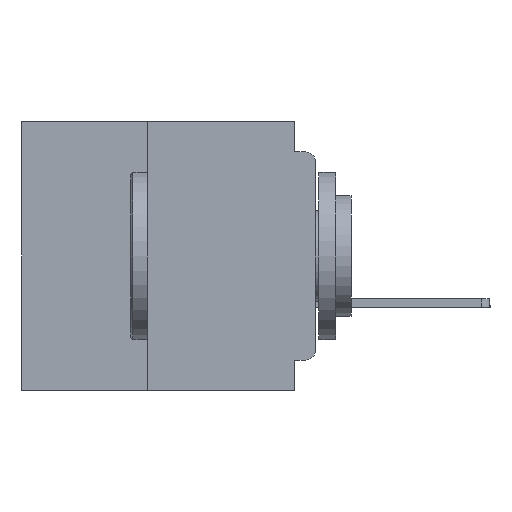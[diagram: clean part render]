
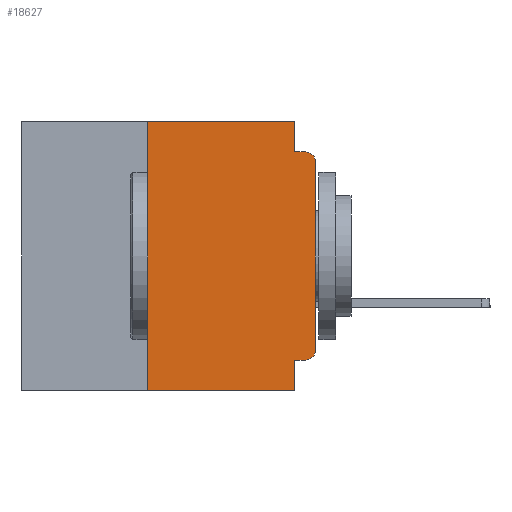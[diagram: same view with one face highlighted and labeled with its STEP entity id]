
A CAD part, left-side view. The second image highlights one B-rep face of the part: STEP entity #18627.
In plain terms, the highlighted planar face has unit normal (-1, 0, 0).
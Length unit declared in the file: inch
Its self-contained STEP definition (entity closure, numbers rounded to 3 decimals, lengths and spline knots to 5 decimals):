
#276 = EDGE_CURVE ( 'NONE', #13432, #35435, #7282, .T. ) ;
#452 = VERTEX_POINT ( 'NONE', #28619 ) ;
#608 = VECTOR ( 'NONE', #24151, 39.37008 ) ;
#1027 = DIRECTION ( 'NONE',  ( 0., 0., -1. ) ) ;
#1033 = CARTESIAN_POINT ( 'NONE',  ( 0., 0.031, -0.355 ) ) ;
#1709 = CARTESIAN_POINT ( 'NONE',  ( 0., 0.031, 0. ) ) ;
#1861 = DIRECTION ( 'NONE',  ( 0., 0., -1. ) ) ;
#2260 = CARTESIAN_POINT ( 'NONE',  ( 0., 0.031, -0.4 ) ) ;
#2428 = VECTOR ( 'NONE', #19470, 39.37008 ) ;
#3715 = CARTESIAN_POINT ( 'NONE',  ( 0., 0.031, 0. ) ) ;
#4009 = LINE ( 'NONE', #33039, #11389 ) ;
#4028 = CIRCLE ( 'NONE', #7651, 0.015 ) ;
#4280 = ORIENTED_EDGE ( 'NONE', *, *, #9184, .T. ) ;
#4414 = VERTEX_POINT ( 'NONE', #18378 ) ;
#5037 = ORIENTED_EDGE ( 'NONE', *, *, #34478, .F. ) ;
#5732 = VECTOR ( 'NONE', #16223, 39.37008 ) ;
#5984 = CARTESIAN_POINT ( 'NONE',  ( 0., 0.015, -0.06 ) ) ;
#7025 = FACE_OUTER_BOUND ( 'NONE', #15466, .T. ) ;
#7117 = LINE ( 'NONE', #10163, #608 ) ;
#7175 = VERTEX_POINT ( 'NONE', #1033 ) ;
#7191 = DIRECTION ( 'NONE',  ( 0., -1., 0. ) ) ;
#7282 = LINE ( 'NONE', #1709, #30344 ) ;
#7651 = AXIS2_PLACEMENT_3D ( 'NONE', #35040, #18512, #1861 ) ;
#8563 = ORIENTED_EDGE ( 'NONE', *, *, #30683, .T. ) ;
#8800 = DIRECTION ( 'NONE',  ( 0., 0., -1. ) ) ;
#8905 = CARTESIAN_POINT ( 'NONE',  ( 0., 0.25, 0. ) ) ;
#9120 = EDGE_CURVE ( 'NONE', #33688, #452, #34362, .T. ) ;
#9158 = EDGE_CURVE ( 'NONE', #35435, #24258, #26239, .T. ) ;
#9184 = EDGE_CURVE ( 'NONE', #33331, #33688, #4028, .T. ) ;
#9328 = PLANE ( 'NONE',  #16297 ) ;
#10163 = CARTESIAN_POINT ( 'NONE',  ( 0., 0., -0.355 ) ) ;
#10335 = AXIS2_PLACEMENT_3D ( 'NONE', #5984, #25486, #8800 ) ;
#10351 = ORIENTED_EDGE ( 'NONE', *, *, #21528, .F. ) ;
#11389 = VECTOR ( 'NONE', #22030, 39.37008 ) ;
#11803 = ORIENTED_EDGE ( 'NONE', *, *, #9120, .T. ) ;
#12261 = ORIENTED_EDGE ( 'NONE', *, *, #22802, .T. ) ;
#12277 = VECTOR ( 'NONE', #7191, 39.37008 ) ;
#12661 = CARTESIAN_POINT ( 'NONE',  ( 0., 0., 0. ) ) ;
#13092 = CARTESIAN_POINT ( 'NONE',  ( 0., 0.031, -0.045 ) ) ;
#13432 = VERTEX_POINT ( 'NONE', #3715 ) ;
#14575 = VERTEX_POINT ( 'NONE', #30294 ) ;
#14913 = DIRECTION ( 'NONE',  ( 1., 0., 0. ) ) ;
#15466 = EDGE_LOOP ( 'NONE', ( #11803, #12261, #21797, #28809, #5037, #20275, #8563, #17272, #10351, #4280 ) ) ;
#16223 = DIRECTION ( 'NONE',  ( 0., 0., -1. ) ) ;
#16297 = AXIS2_PLACEMENT_3D ( 'NONE', #28794, #14913, #34265 ) ;
#16672 = CARTESIAN_POINT ( 'NONE',  ( 0., 0.437, 0. ) ) ;
#17272 = ORIENTED_EDGE ( 'NONE', *, *, #22589, .F. ) ;
#18378 = CARTESIAN_POINT ( 'NONE',  ( 0., 0.25, -0.4 ) ) ;
#18385 = CARTESIAN_POINT ( 'NONE',  ( 0., 0., -0.045 ) ) ;
#18512 = DIRECTION ( 'NONE',  ( -1., 0., 0. ) ) ;
#18627 = ADVANCED_FACE ( 'NONE', ( #7025 ), #9328, .F. ) ;
#19470 = DIRECTION ( 'NONE',  ( 0., -1., 0. ) ) ;
#20275 = ORIENTED_EDGE ( 'NONE', *, *, #22684, .F. ) ;
#20718 = CARTESIAN_POINT ( 'NONE',  ( 0., 0.015, -0.045 ) ) ;
#20985 = CARTESIAN_POINT ( 'NONE',  ( 0., 0.437, -0.4 ) ) ;
#21100 = DIRECTION ( 'NONE',  ( 0., -1., 0. ) ) ;
#21391 = VECTOR ( 'NONE', #21100, 39.37008 ) ;
#21528 = EDGE_CURVE ( 'NONE', #33331, #7175, #7117, .T. ) ;
#21797 = ORIENTED_EDGE ( 'NONE', *, *, #9158, .F. ) ;
#22030 = DIRECTION ( 'NONE',  ( 0., 0., 1. ) ) ;
#22589 = EDGE_CURVE ( 'NONE', #7175, #14575, #27951, .T. ) ;
#22684 = EDGE_CURVE ( 'NONE', #4414, #26399, #4009, .T. ) ;
#22802 = EDGE_CURVE ( 'NONE', #452, #24258, #28359, .T. ) ;
#24151 = DIRECTION ( 'NONE',  ( 0., 1., 0. ) ) ;
#24258 = VERTEX_POINT ( 'NONE', #20718 ) ;
#25486 = DIRECTION ( 'NONE',  ( -1., 0., 0. ) ) ;
#25508 = LINE ( 'NONE', #16672, #2428 ) ;
#26239 = LINE ( 'NONE', #18385, #12277 ) ;
#26399 = VERTEX_POINT ( 'NONE', #8905 ) ;
#27112 = CARTESIAN_POINT ( 'NONE',  ( 0., 0., -0.34 ) ) ;
#27951 = LINE ( 'NONE', #2260, #5732 ) ;
#28359 = CIRCLE ( 'NONE', #10335, 0.015 ) ;
#28619 = CARTESIAN_POINT ( 'NONE',  ( 0., 0., -0.06 ) ) ;
#28794 = CARTESIAN_POINT ( 'NONE',  ( 0., 0.437, 0. ) ) ;
#28809 = ORIENTED_EDGE ( 'NONE', *, *, #276, .F. ) ;
#28820 = LINE ( 'NONE', #20985, #21391 ) ;
#30294 = CARTESIAN_POINT ( 'NONE',  ( 0., 0.031, -0.4 ) ) ;
#30344 = VECTOR ( 'NONE', #1027, 39.37008 ) ;
#30683 = EDGE_CURVE ( 'NONE', #4414, #14575, #28820, .T. ) ;
#32073 = DIRECTION ( 'NONE',  ( 0., 0., 1. ) ) ;
#32833 = CARTESIAN_POINT ( 'NONE',  ( 0., 0.015, -0.355 ) ) ;
#33039 = CARTESIAN_POINT ( 'NONE',  ( 0., 0.25, -0.4 ) ) ;
#33331 = VERTEX_POINT ( 'NONE', #32833 ) ;
#33688 = VERTEX_POINT ( 'NONE', #27112 ) ;
#34265 = DIRECTION ( 'NONE',  ( 0., 0., -1. ) ) ;
#34362 = LINE ( 'NONE', #12661, #35225 ) ;
#34478 = EDGE_CURVE ( 'NONE', #26399, #13432, #25508, .T. ) ;
#35040 = CARTESIAN_POINT ( 'NONE',  ( 0., 0.015, -0.34 ) ) ;
#35225 = VECTOR ( 'NONE', #32073, 39.37008 ) ;
#35435 = VERTEX_POINT ( 'NONE', #13092 ) ;
